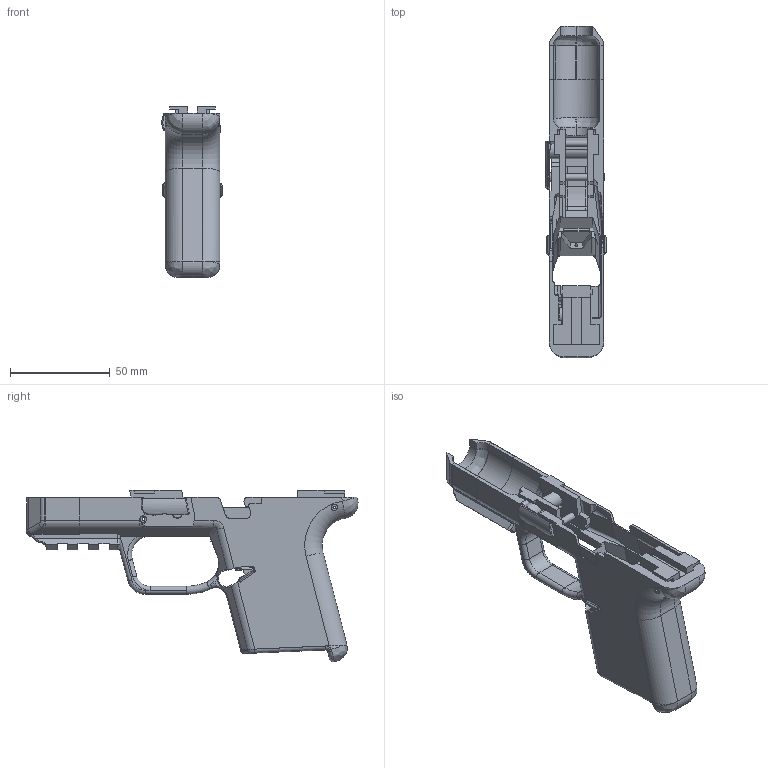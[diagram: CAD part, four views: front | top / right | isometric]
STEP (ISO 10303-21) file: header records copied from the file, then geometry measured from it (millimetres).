
FILE_DESCRIPTION(/* description */ (''),/* implementation_level */ '2;1');
FILE_NAME(/* name */ 'M&P 9 Assembly + Picatinny - Compact Length Slide.step',/* time_stamp */ '2022-02-26T19:53:04-05:00',/* author */ (''),/* organization */ (''),/* preprocessor_version */ 'ST-DEVELOPER v18.1',/* originating_system */ 'Autodesk Translation Framework v10.13.0.1454',/* authorisation */ '');
FILE_SCHEMA (('AUTOMOTIVE_DESIGN { 1 0 10303 214 3 1 1 }'));
Length unit declared in the file: millimetre
Products named in the file (11): M&P 9 Compact Length Slide - Picatinny; M&P 9 Reference v117; Rear Fire Control Group Pin; Front Locking Block Group Pin; Trigger Pin; Locking Block; Disassembly Lug; Rear Fire Control Group; Frame; Fitment Section; M1.0 Full-size Nose
Assembly tree (10 placements, depth 5):
  M&P 9 Compact Length Slide - Picatinny
    M&P 9 Reference v117
      Rear Fire Control Group Pin
      Front Locking Block Group Pin
      Trigger Pin
      Locking Block
      Disassembly Lug
      Rear Fire Control Group
      Frame
        Fitment Section
          M1.0 Full-size Nose
Bounding box: 30.21 x 166.61 x 86.03 mm (x, y, z)
Volume: 85324.9 mm3; surface area: 50084.2 mm2
Topology: 12 solids, 12 shells, 642 faces, 1749 edges, 1121 vertices
Faces by surface type: plane 348, cylinder 184, bspline 83, torus 21, sphere 4, cone 2
Full cylindrical faces by diameter (mm): 1.35 x2, 1.5 x2, 3.15 x2, 3.18 x3, 3.2 x2, 3.361 x2, 3.5 x1, 3.55 x4, 4.7 x1, 5.1 x1, 6.3 x1, 7.7 x1, 8.8 x1, 9 x2
Entity records: 23529 total; most frequent: CARTESIAN_POINT 7136, ORIENTED_EDGE 3490, DIRECTION 3203, EDGE_CURVE 1745, VERTEX_POINT 1121, LINE 1097, VECTOR 1097, AXIS2_PLACEMENT_3D 1053
